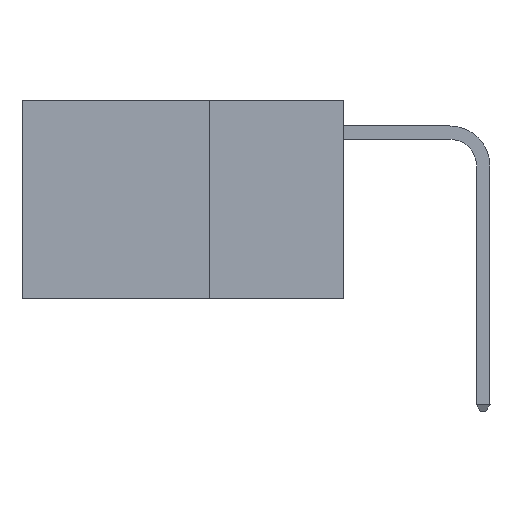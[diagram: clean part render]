
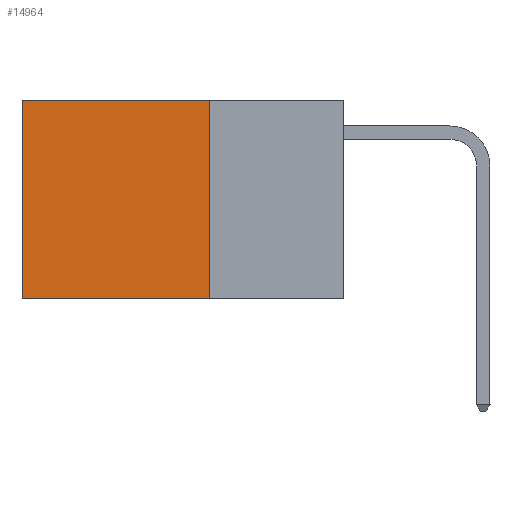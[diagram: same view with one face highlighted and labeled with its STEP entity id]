
A CAD part, left-side view. The second image highlights one B-rep face of the part: STEP entity #14964.
In plain terms, the highlighted planar face has unit normal (-1, 0, 0).
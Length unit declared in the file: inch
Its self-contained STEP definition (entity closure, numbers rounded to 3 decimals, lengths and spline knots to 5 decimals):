
#805 = DIRECTION ( 'NONE',  ( 1., 0., 0. ) ) ;
#1355 = EDGE_CURVE ( 'NONE', #13697, #11956, #16555, .T. ) ;
#2238 = VECTOR ( 'NONE', #9333, 39.37008 ) ;
#2354 = EDGE_CURVE ( 'NONE', #8044, #11207, #12622, .T. ) ;
#2388 = VECTOR ( 'NONE', #4739, 39.37008 ) ;
#3421 = CARTESIAN_POINT ( 'NONE',  ( 0.2625, 0.25, 0. ) ) ;
#4562 = DIRECTION ( 'NONE',  ( 0., 1., 0. ) ) ;
#4739 = DIRECTION ( 'NONE',  ( 0., 0., -1. ) ) ;
#5436 = DIRECTION ( 'NONE',  ( 0., 0., -1. ) ) ;
#5623 = AXIS2_PLACEMENT_3D ( 'NONE', #8640, #805, #10004 ) ;
#6226 = VECTOR ( 'NONE', #4562, 39.37008 ) ;
#6374 = VECTOR ( 'NONE', #5436, 39.37008 ) ;
#7104 = CARTESIAN_POINT ( 'NONE',  ( 0.2625, 0.25, -0.37 ) ) ;
#7166 = EDGE_CURVE ( 'NONE', #11956, #11207, #16960, .T. ) ;
#7352 = ORIENTED_EDGE ( 'NONE', *, *, #7166, .F. ) ;
#7993 = CARTESIAN_POINT ( 'NONE',  ( 0.2625, 0.25, 0. ) ) ;
#8044 = VERTEX_POINT ( 'NONE', #16999 ) ;
#8640 = CARTESIAN_POINT ( 'NONE',  ( 0.2625, 0.25, 0. ) ) ;
#9011 = CARTESIAN_POINT ( 'NONE',  ( 0.2625, 0.25, -0.37 ) ) ;
#9328 = ORIENTED_EDGE ( 'NONE', *, *, #2354, .T. ) ;
#9333 = DIRECTION ( 'NONE',  ( 0., 1., 0. ) ) ;
#9368 = CARTESIAN_POINT ( 'NONE',  ( 0.2625, 0.6, 0. ) ) ;
#9947 = PLANE ( 'NONE',  #5623 ) ;
#10004 = DIRECTION ( 'NONE',  ( 0., 0., -1. ) ) ;
#10235 = ORIENTED_EDGE ( 'NONE', *, *, #1355, .F. ) ;
#11077 = FACE_OUTER_BOUND ( 'NONE', #14790, .T. ) ;
#11207 = VERTEX_POINT ( 'NONE', #11570 ) ;
#11570 = CARTESIAN_POINT ( 'NONE',  ( 0.2625, 0.6, -0.37 ) ) ;
#11956 = VERTEX_POINT ( 'NONE', #9011 ) ;
#12520 = CARTESIAN_POINT ( 'NONE',  ( 0.2625, 0.25, 0. ) ) ;
#12622 = LINE ( 'NONE', #9368, #6374 ) ;
#12768 = LINE ( 'NONE', #7993, #2238 ) ;
#13697 = VERTEX_POINT ( 'NONE', #12520 ) ;
#14759 = ORIENTED_EDGE ( 'NONE', *, *, #15298, .T. ) ;
#14790 = EDGE_LOOP ( 'NONE', ( #9328, #7352, #10235, #14759 ) ) ;
#14964 = ADVANCED_FACE ( 'NONE', ( #11077 ), #9947, .F. ) ;
#15298 = EDGE_CURVE ( 'NONE', #13697, #8044, #12768, .T. ) ;
#16555 = LINE ( 'NONE', #3421, #2388 ) ;
#16960 = LINE ( 'NONE', #7104, #6226 ) ;
#16999 = CARTESIAN_POINT ( 'NONE',  ( 0.2625, 0.6, 0. ) ) ;
